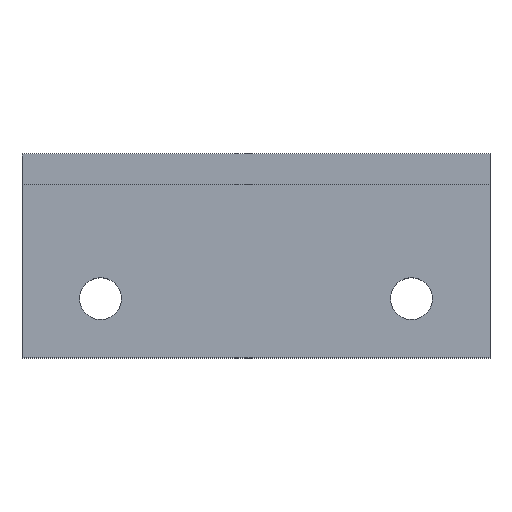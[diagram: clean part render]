
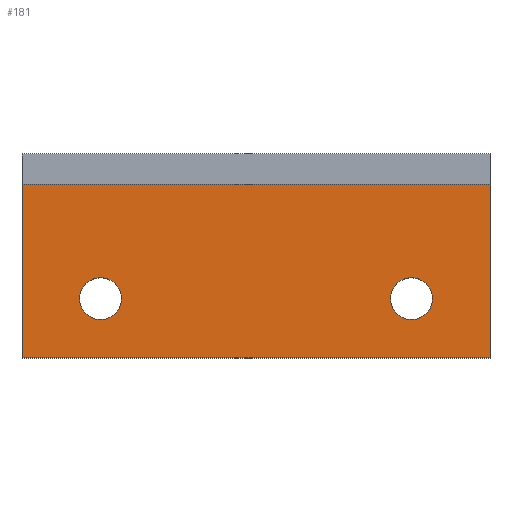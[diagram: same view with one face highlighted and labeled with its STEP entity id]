
A CAD part, top view. The second image highlights one B-rep face of the part: STEP entity #181.
In plain terms, the highlighted planar face has unit normal (0, 0, 1).
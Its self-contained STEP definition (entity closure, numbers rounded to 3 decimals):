
#15=LINE('',#285,#33);
#16=LINE('',#287,#34);
#17=LINE('',#289,#35);
#18=LINE('',#290,#36);
#33=VECTOR('',#239,10.);
#34=VECTOR('',#240,10.);
#35=VECTOR('',#241,10.);
#36=VECTOR('',#242,10.);
#51=PLANE('',#215);
#61=FACE_BOUND('',#80,.T.);
#62=FACE_BOUND('',#81,.T.);
#67=FACE_OUTER_BOUND('',#79,.T.);
#79=EDGE_LOOP('',(#137,#138,#139,#140));
#80=EDGE_LOOP('',(#141));
#81=EDGE_LOOP('',(#142));
#92=CIRCLE('',#211,0.8);
#94=CIRCLE('',#214,0.8);
#96=VERTEX_POINT('',#275);
#98=VERTEX_POINT('',#280);
#99=VERTEX_POINT('',#283);
#100=VERTEX_POINT('',#284);
#101=VERTEX_POINT('',#286);
#102=VERTEX_POINT('',#288);
#112=EDGE_CURVE('',#96,#96,#92,.T.);
#114=EDGE_CURVE('',#98,#98,#94,.T.);
#115=EDGE_CURVE('',#99,#100,#15,.T.);
#116=EDGE_CURVE('',#101,#100,#16,.T.);
#117=EDGE_CURVE('',#102,#101,#17,.T.);
#118=EDGE_CURVE('',#99,#102,#18,.T.);
#137=ORIENTED_EDGE('',*,*,#115,.T.);
#138=ORIENTED_EDGE('',*,*,#116,.F.);
#139=ORIENTED_EDGE('',*,*,#117,.F.);
#140=ORIENTED_EDGE('',*,*,#118,.F.);
#141=ORIENTED_EDGE('',*,*,#112,.T.);
#142=ORIENTED_EDGE('',*,*,#114,.T.);
#181=ADVANCED_FACE('',(#67,#61,#62),#51,.F.);
#211=AXIS2_PLACEMENT_3D('',#276,#229,#230);
#214=AXIS2_PLACEMENT_3D('',#281,#235,#236);
#215=AXIS2_PLACEMENT_3D('',#282,#237,#238);
#229=DIRECTION('center_axis',(0.,0.,-1.));
#230=DIRECTION('ref_axis',(-1.,0.,0.));
#235=DIRECTION('center_axis',(0.,0.,-1.));
#236=DIRECTION('ref_axis',(-1.,0.,0.));
#237=DIRECTION('center_axis',(0.,0.,-1.));
#238=DIRECTION('ref_axis',(0.,1.,0.));
#239=DIRECTION('',(-1.,0.,0.));
#240=DIRECTION('',(0.,1.,0.));
#241=DIRECTION('',(-1.,0.,0.));
#242=DIRECTION('',(0.,-1.,0.));
#275=CARTESIAN_POINT('',(17.8,-3.522,10.036));
#276=CARTESIAN_POINT('Origin',(17.,-3.522,10.036));
#280=CARTESIAN_POINT('',(5.934,-3.522,10.036));
#281=CARTESIAN_POINT('Origin',(5.134,-3.522,10.036));
#282=CARTESIAN_POINT('Origin',(0.,-1.,10.036));
#283=CARTESIAN_POINT('',(20.,0.84,10.036));
#284=CARTESIAN_POINT('',(2.134,0.84,10.036));
#285=CARTESIAN_POINT('',(0.,0.84,10.036));
#286=CARTESIAN_POINT('',(2.134,-5.782,10.036));
#287=CARTESIAN_POINT('',(2.134,0.75,10.036));
#288=CARTESIAN_POINT('',(20.,-5.782,10.036));
#289=CARTESIAN_POINT('',(7.595,-5.782,10.036));
#290=CARTESIAN_POINT('',(20.,-3.391,10.036));
